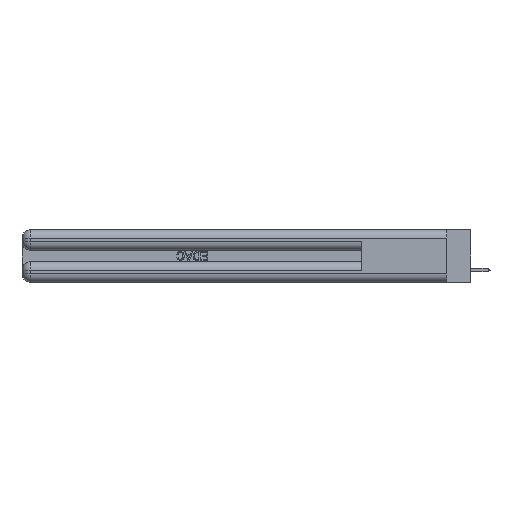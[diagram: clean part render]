
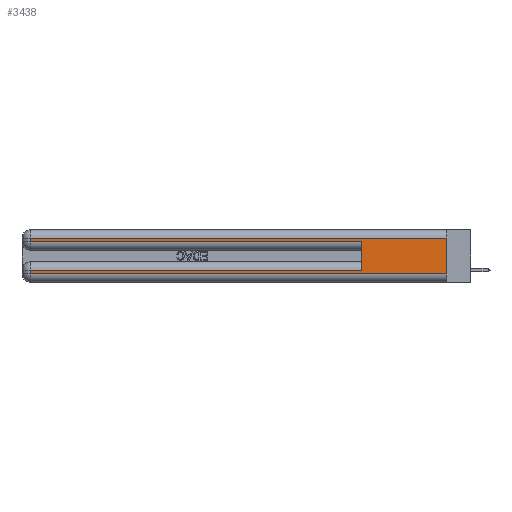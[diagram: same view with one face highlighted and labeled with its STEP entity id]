
A CAD part, left-side view. The second image highlights one B-rep face of the part: STEP entity #3438.
In plain terms, the highlighted planar face has unit normal (-1, 0, 0).
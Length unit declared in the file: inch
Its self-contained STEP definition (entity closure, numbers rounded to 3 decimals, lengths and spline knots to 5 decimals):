
#373 = DIRECTION ( 'NONE',  ( 0., -1., 0. ) ) ;
#1377 = CARTESIAN_POINT ( 'NONE',  ( 0., 0., 0.06 ) ) ;
#1574 = DIRECTION ( 'NONE',  ( 0., 1., 0. ) ) ;
#2576 = ORIENTED_EDGE ( 'NONE', *, *, #29415, .F. ) ;
#3438 = ADVANCED_FACE ( 'NONE', ( #7544 ), #37332, .F. ) ;
#4394 = DIRECTION ( 'NONE',  ( 0., 1., 0. ) ) ;
#4473 = CARTESIAN_POINT ( 'NONE',  ( 0., 2.94, 0.285 ) ) ;
#5786 = VECTOR ( 'NONE', #29118, 39.37008 ) ;
#6000 = ORIENTED_EDGE ( 'NONE', *, *, #26453, .T. ) ;
#6238 = VECTOR ( 'NONE', #1574, 39.37008 ) ;
#6677 = EDGE_CURVE ( 'NONE', #30813, #16589, #15385, .T. ) ;
#7384 = CARTESIAN_POINT ( 'NONE',  ( 0., 0., 0.085 ) ) ;
#7522 = VERTEX_POINT ( 'NONE', #4473 ) ;
#7544 = FACE_OUTER_BOUND ( 'NONE', #30966, .T. ) ;
#7734 = LINE ( 'NONE', #21075, #19086 ) ;
#8641 = VECTOR ( 'NONE', #36792, 39.37008 ) ;
#9142 = VECTOR ( 'NONE', #9743, 39.37008 ) ;
#9743 = DIRECTION ( 'NONE',  ( 0., -1., 0. ) ) ;
#11645 = VECTOR ( 'NONE', #35744, 39.37008 ) ;
#13881 = CARTESIAN_POINT ( 'NONE',  ( 0., 2.94, 0.06 ) ) ;
#14192 = VERTEX_POINT ( 'NONE', #16246 ) ;
#15164 = CARTESIAN_POINT ( 'NONE',  ( 0., 0., 0.31 ) ) ;
#15241 = VERTEX_POINT ( 'NONE', #23094 ) ;
#15385 = LINE ( 'NONE', #7384, #6238 ) ;
#16246 = CARTESIAN_POINT ( 'NONE',  ( 0., 0.6, 0.285 ) ) ;
#16589 = VERTEX_POINT ( 'NONE', #24735 ) ;
#17086 = LINE ( 'NONE', #33487, #11645 ) ;
#17323 = CARTESIAN_POINT ( 'NONE',  ( 0., 0., 0.37 ) ) ;
#19019 = LINE ( 'NONE', #30172, #26750 ) ;
#19086 = VECTOR ( 'NONE', #26377, 39.37008 ) ;
#19463 = VECTOR ( 'NONE', #373, 39.37008 ) ;
#19874 = DIRECTION ( 'NONE',  ( 1., 0., 0. ) ) ;
#20584 = ORIENTED_EDGE ( 'NONE', *, *, #6677, .T. ) ;
#21075 = CARTESIAN_POINT ( 'NONE',  ( 0., 0., 0.37 ) ) ;
#21081 = CARTESIAN_POINT ( 'NONE',  ( 0., 0., 0.285 ) ) ;
#22425 = CARTESIAN_POINT ( 'NONE',  ( 0., 0.6, 0.145 ) ) ;
#22502 = ORIENTED_EDGE ( 'NONE', *, *, #30291, .T. ) ;
#22734 = EDGE_CURVE ( 'NONE', #7522, #14192, #34856, .T. ) ;
#22946 = DIRECTION ( 'NONE',  ( 0., 0., -1. ) ) ;
#23094 = CARTESIAN_POINT ( 'NONE',  ( 0., 2.94, 0.31 ) ) ;
#23199 = ORIENTED_EDGE ( 'NONE', *, *, #27860, .T. ) ;
#23766 = VERTEX_POINT ( 'NONE', #13881 ) ;
#24126 = EDGE_CURVE ( 'NONE', #15241, #7522, #17086, .T. ) ;
#24735 = CARTESIAN_POINT ( 'NONE',  ( 0., 2.94, 0.085 ) ) ;
#25138 = VERTEX_POINT ( 'NONE', #29391 ) ;
#25492 = LINE ( 'NONE', #36166, #8641 ) ;
#26377 = DIRECTION ( 'NONE',  ( 0., 0., -1. ) ) ;
#26453 = EDGE_CURVE ( 'NONE', #23766, #25138, #33673, .T. ) ;
#26750 = VECTOR ( 'NONE', #4394, 39.37008 ) ;
#27860 = EDGE_CURVE ( 'NONE', #16589, #23766, #25492, .T. ) ;
#29118 = DIRECTION ( 'NONE',  ( 0., 0., 1. ) ) ;
#29391 = CARTESIAN_POINT ( 'NONE',  ( 0., 0., 0.06 ) ) ;
#29415 = EDGE_CURVE ( 'NONE', #30813, #14192, #31692, .T. ) ;
#30034 = EDGE_CURVE ( 'NONE', #37573, #25138, #7734, .T. ) ;
#30172 = CARTESIAN_POINT ( 'NONE',  ( 0., 0., 0.31 ) ) ;
#30291 = EDGE_CURVE ( 'NONE', #37573, #15241, #19019, .T. ) ;
#30813 = VERTEX_POINT ( 'NONE', #31915 ) ;
#30966 = EDGE_LOOP ( 'NONE', ( #33057, #22502, #35615, #35281, #2576, #20584, #23199, #6000 ) ) ;
#31692 = LINE ( 'NONE', #22425, #5786 ) ;
#31915 = CARTESIAN_POINT ( 'NONE',  ( 0., 0.6, 0.085 ) ) ;
#33057 = ORIENTED_EDGE ( 'NONE', *, *, #30034, .F. ) ;
#33487 = CARTESIAN_POINT ( 'NONE',  ( 0., 2.94, 0.37 ) ) ;
#33673 = LINE ( 'NONE', #1377, #9142 ) ;
#33676 = AXIS2_PLACEMENT_3D ( 'NONE', #17323, #19874, #22946 ) ;
#34856 = LINE ( 'NONE', #21081, #19463 ) ;
#35281 = ORIENTED_EDGE ( 'NONE', *, *, #22734, .T. ) ;
#35615 = ORIENTED_EDGE ( 'NONE', *, *, #24126, .T. ) ;
#35744 = DIRECTION ( 'NONE',  ( 0., 0., -1. ) ) ;
#36166 = CARTESIAN_POINT ( 'NONE',  ( 0., 2.94, 0.37 ) ) ;
#36792 = DIRECTION ( 'NONE',  ( 0., 0., -1. ) ) ;
#37332 = PLANE ( 'NONE',  #33676 ) ;
#37573 = VERTEX_POINT ( 'NONE', #15164 ) ;
